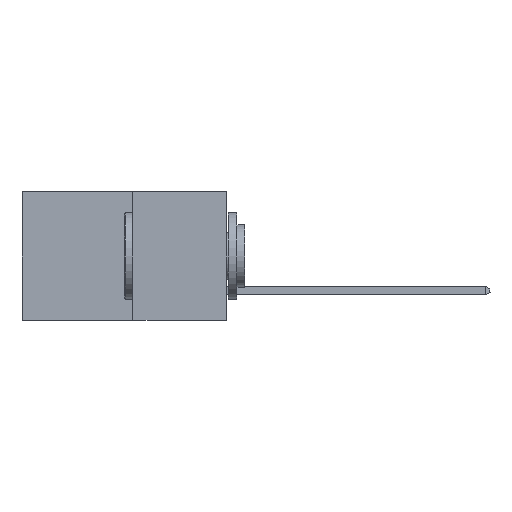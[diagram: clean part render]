
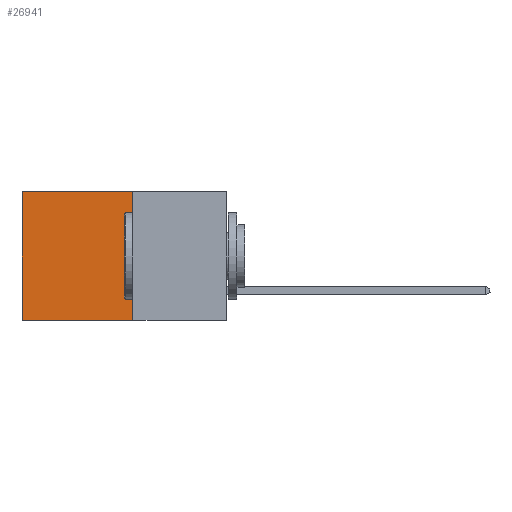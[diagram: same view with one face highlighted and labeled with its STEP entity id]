
A CAD part, left-side view. The second image highlights one B-rep face of the part: STEP entity #26941.
In plain terms, the highlighted planar face has unit normal (-1, 0, 0).
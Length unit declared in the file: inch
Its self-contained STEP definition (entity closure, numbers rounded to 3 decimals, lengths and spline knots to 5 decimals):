
#891 = VECTOR ( 'NONE', #5204, 39.37008 ) ;
#1288 = CARTESIAN_POINT ( 'NONE',  ( 0.277, 0.59, 0. ) ) ;
#2512 = LINE ( 'NONE', #10457, #891 ) ;
#2842 = EDGE_LOOP ( 'NONE', ( #10206, #25035, #4390, #30955 ) ) ;
#3947 = CARTESIAN_POINT ( 'NONE',  ( 0.277, 0.27, -0.37 ) ) ;
#4390 = ORIENTED_EDGE ( 'NONE', *, *, #32357, .F. ) ;
#5024 = CARTESIAN_POINT ( 'NONE',  ( 0.277, 0.59, -0.37 ) ) ;
#5204 = DIRECTION ( 'NONE',  ( 0., 1., 0. ) ) ;
#5251 = FACE_OUTER_BOUND ( 'NONE', #2842, .T. ) ;
#5360 = LINE ( 'NONE', #18787, #11492 ) ;
#6981 = EDGE_CURVE ( 'NONE', #15257, #7790, #21747, .T. ) ;
#7336 = LINE ( 'NONE', #24215, #12644 ) ;
#7790 = VERTEX_POINT ( 'NONE', #5024 ) ;
#7902 = VECTOR ( 'NONE', #19133, 39.37008 ) ;
#8045 = CARTESIAN_POINT ( 'NONE',  ( 0.277, 0.27, 0. ) ) ;
#8679 = EDGE_CURVE ( 'NONE', #13159, #7790, #2512, .T. ) ;
#9108 = AXIS2_PLACEMENT_3D ( 'NONE', #3947, #19525, #14440 ) ;
#9173 = PLANE ( 'NONE',  #9108 ) ;
#10206 = ORIENTED_EDGE ( 'NONE', *, *, #6981, .T. ) ;
#10457 = CARTESIAN_POINT ( 'NONE',  ( 0.277, 0.27, -0.37 ) ) ;
#10752 = VERTEX_POINT ( 'NONE', #8045 ) ;
#11374 = DIRECTION ( 'NONE',  ( 0., 1., 0. ) ) ;
#11492 = VECTOR ( 'NONE', #26563, 39.37008 ) ;
#12644 = VECTOR ( 'NONE', #11374, 39.37008 ) ;
#13159 = VERTEX_POINT ( 'NONE', #31740 ) ;
#14440 = DIRECTION ( 'NONE',  ( 0., 0., -1. ) ) ;
#15163 = EDGE_CURVE ( 'NONE', #10752, #15257, #7336, .T. ) ;
#15257 = VERTEX_POINT ( 'NONE', #1288 ) ;
#18787 = CARTESIAN_POINT ( 'NONE',  ( 0.277, 0.27, -0.37 ) ) ;
#19133 = DIRECTION ( 'NONE',  ( 0., 0., -1. ) ) ;
#19240 = CARTESIAN_POINT ( 'NONE',  ( 0.277, 0.59, -0.37 ) ) ;
#19525 = DIRECTION ( 'NONE',  ( 1., 0., 0. ) ) ;
#21747 = LINE ( 'NONE', #19240, #7902 ) ;
#24215 = CARTESIAN_POINT ( 'NONE',  ( 0.277, 0.27, 0. ) ) ;
#25035 = ORIENTED_EDGE ( 'NONE', *, *, #8679, .F. ) ;
#26563 = DIRECTION ( 'NONE',  ( 0., 0., -1. ) ) ;
#26941 = ADVANCED_FACE ( 'NONE', ( #5251 ), #9173, .F. ) ;
#30955 = ORIENTED_EDGE ( 'NONE', *, *, #15163, .T. ) ;
#31740 = CARTESIAN_POINT ( 'NONE',  ( 0.277, 0.27, -0.37 ) ) ;
#32357 = EDGE_CURVE ( 'NONE', #10752, #13159, #5360, .T. ) ;
